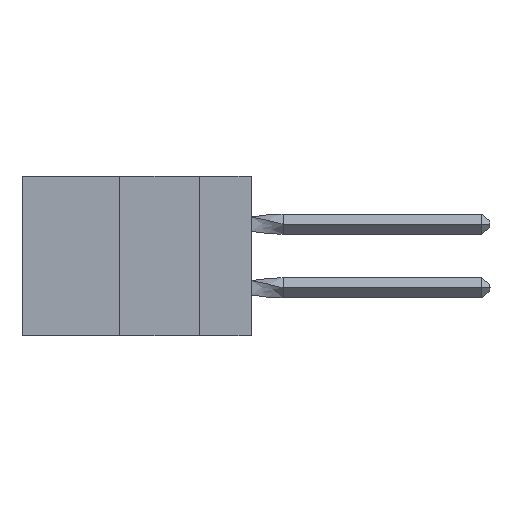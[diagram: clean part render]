
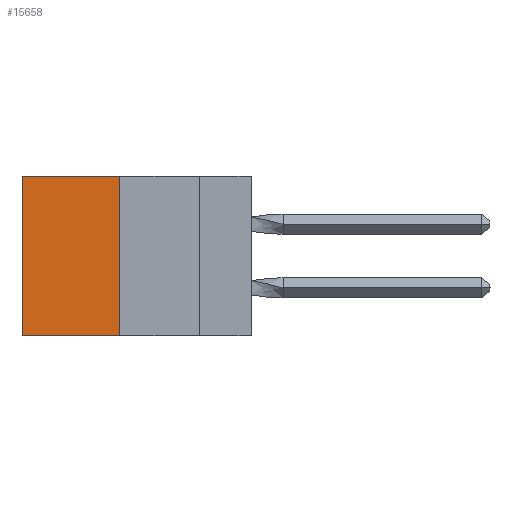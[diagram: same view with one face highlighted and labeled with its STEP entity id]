
A CAD part, left-side view. The second image highlights one B-rep face of the part: STEP entity #15658.
In plain terms, the highlighted planar face has unit normal (-1, 0, 0).
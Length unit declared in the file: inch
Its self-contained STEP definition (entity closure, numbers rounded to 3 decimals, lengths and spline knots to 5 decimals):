
#1078 = CARTESIAN_POINT ( 'NONE',  ( 0.305, 0.72, -0.5 ) ) ;
#1410 = EDGE_CURVE ( 'NONE', #14263, #11121, #15891, .T. ) ;
#2125 = CARTESIAN_POINT ( 'NONE',  ( 0.305, 0.413, -0.5 ) ) ;
#2167 = VECTOR ( 'NONE', #22183, 39.37008 ) ;
#3253 = CARTESIAN_POINT ( 'NONE',  ( 0.305, 0.72, -0.5 ) ) ;
#3523 = CARTESIAN_POINT ( 'NONE',  ( 0.305, 0.413, 0. ) ) ;
#4015 = DIRECTION ( 'NONE',  ( 0., 0., -1. ) ) ;
#4224 = EDGE_CURVE ( 'NONE', #9367, #17434, #10857, .T. ) ;
#4401 = LINE ( 'NONE', #3523, #2167 ) ;
#5031 = DIRECTION ( 'NONE',  ( 0., 0., -1. ) ) ;
#8339 = DIRECTION ( 'NONE',  ( 0., 1., 0. ) ) ;
#9233 = DIRECTION ( 'NONE',  ( 1., 0., 0. ) ) ;
#9367 = VERTEX_POINT ( 'NONE', #15210 ) ;
#10857 = LINE ( 'NONE', #2125, #20525 ) ;
#11121 = VERTEX_POINT ( 'NONE', #3253 ) ;
#11123 = CARTESIAN_POINT ( 'NONE',  ( 0.305, 0.413, -0.5 ) ) ;
#11690 = VECTOR ( 'NONE', #5031, 39.37008 ) ;
#11973 = ORIENTED_EDGE ( 'NONE', *, *, #1410, .T. ) ;
#13151 = EDGE_LOOP ( 'NONE', ( #11973, #26582, #25019, #25788 ) ) ;
#14263 = VERTEX_POINT ( 'NONE', #18968 ) ;
#14449 = CARTESIAN_POINT ( 'NONE',  ( 0.305, 0.413, -0.5 ) ) ;
#15190 = DIRECTION ( 'NONE',  ( 0., 0., -1. ) ) ;
#15210 = CARTESIAN_POINT ( 'NONE',  ( 0.305, 0.413, 0. ) ) ;
#15273 = PLANE ( 'NONE',  #21346 ) ;
#15658 = ADVANCED_FACE ( 'NONE', ( #18469 ), #15273, .F. ) ;
#15891 = LINE ( 'NONE', #1078, #11690 ) ;
#17434 = VERTEX_POINT ( 'NONE', #22533 ) ;
#18444 = EDGE_CURVE ( 'NONE', #17434, #11121, #26644, .T. ) ;
#18469 = FACE_OUTER_BOUND ( 'NONE', #13151, .T. ) ;
#18968 = CARTESIAN_POINT ( 'NONE',  ( 0.305, 0.72, 0. ) ) ;
#20525 = VECTOR ( 'NONE', #4015, 39.37008 ) ;
#21253 = VECTOR ( 'NONE', #8339, 39.37008 ) ;
#21346 = AXIS2_PLACEMENT_3D ( 'NONE', #11123, #9233, #15190 ) ;
#22183 = DIRECTION ( 'NONE',  ( 0., 1., 0. ) ) ;
#22533 = CARTESIAN_POINT ( 'NONE',  ( 0.305, 0.413, -0.5 ) ) ;
#24429 = EDGE_CURVE ( 'NONE', #9367, #14263, #4401, .T. ) ;
#25019 = ORIENTED_EDGE ( 'NONE', *, *, #4224, .F. ) ;
#25788 = ORIENTED_EDGE ( 'NONE', *, *, #24429, .T. ) ;
#26582 = ORIENTED_EDGE ( 'NONE', *, *, #18444, .F. ) ;
#26644 = LINE ( 'NONE', #14449, #21253 ) ;
